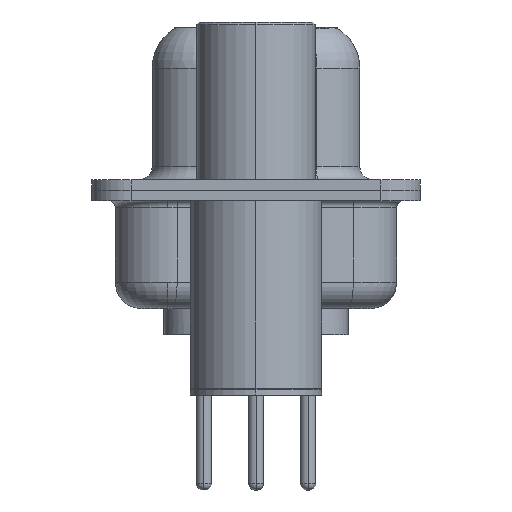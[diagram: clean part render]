
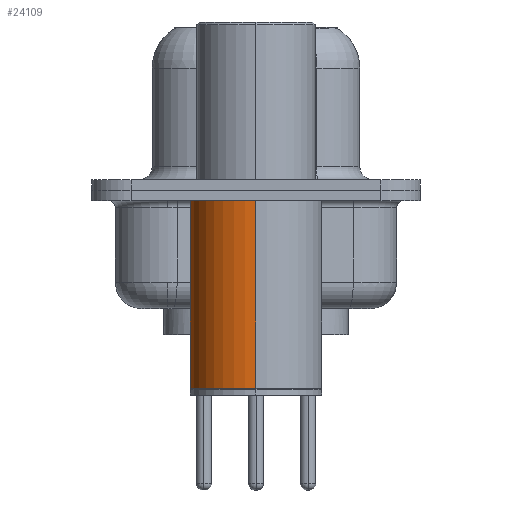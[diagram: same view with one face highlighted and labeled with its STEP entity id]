
A CAD part, left-side view. The second image highlights one B-rep face of the part: STEP entity #24109.
In plain terms, the highlighted cylindrical face has radius 2.5 mm (diameter 5 mm), a partial arc.
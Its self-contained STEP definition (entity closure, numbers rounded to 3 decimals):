
#884 = EDGE_CURVE ( 'NONE', #31840, #3143, #14207, .T. ) ;
#1985 = ORIENTED_EDGE ( 'NONE', *, *, #25627, .T. ) ;
#2144 = VECTOR ( 'NONE', #2211, 1000. ) ;
#2211 = DIRECTION ( 'NONE',  ( 0., 0., 1. ) ) ;
#2372 = CARTESIAN_POINT ( 'NONE',  ( 2.5, 0., -7.525 ) ) ;
#3133 = VERTEX_POINT ( 'NONE', #2372 ) ;
#3143 = VERTEX_POINT ( 'NONE', #9293 ) ;
#4476 = DIRECTION ( 'NONE',  ( 1., 0., 0. ) ) ;
#4681 = DIRECTION ( 'NONE',  ( 1., 0., 0. ) ) ;
#7288 = VERTEX_POINT ( 'NONE', #30706 ) ;
#7752 = ORIENTED_EDGE ( 'NONE', *, *, #14204, .F. ) ;
#8628 = LINE ( 'NONE', #18679, #12367 ) ;
#9293 = CARTESIAN_POINT ( 'NONE',  ( -2.5, 0., -0.4 ) ) ;
#11117 = CARTESIAN_POINT ( 'NONE',  ( 0., 0., 0.581 ) ) ;
#12092 = DIRECTION ( 'NONE',  ( 0., 0., 1. ) ) ;
#12190 = CIRCLE ( 'NONE', #21144, 2.5 ) ;
#12367 = VECTOR ( 'NONE', #31345, 1000. ) ;
#12710 = AXIS2_PLACEMENT_3D ( 'NONE', #11117, #24132, #16705 ) ;
#13914 = CYLINDRICAL_SURFACE ( 'NONE', #12710, 2.5 ) ;
#14204 = EDGE_CURVE ( 'NONE', #3133, #31840, #27725, .T. ) ;
#14207 = CIRCLE ( 'NONE', #16828, 2.5 ) ;
#16705 = DIRECTION ( 'NONE',  ( 1., 0., 0. ) ) ;
#16828 = AXIS2_PLACEMENT_3D ( 'NONE', #21594, #22099, #4476 ) ;
#18679 = CARTESIAN_POINT ( 'NONE',  ( -2.5, 0., 0.581 ) ) ;
#21144 = AXIS2_PLACEMENT_3D ( 'NONE', #29698, #12092, #4681 ) ;
#21594 = CARTESIAN_POINT ( 'NONE',  ( 0., 0., -0.4 ) ) ;
#22099 = DIRECTION ( 'NONE',  ( 0., 0., 1. ) ) ;
#23635 = FACE_OUTER_BOUND ( 'NONE', #29499, .T. ) ;
#24109 = ADVANCED_FACE ( 'NONE', ( #23635 ), #13914, .T. ) ;
#24132 = DIRECTION ( 'NONE',  ( 0., 0., 1. ) ) ;
#24938 = CARTESIAN_POINT ( 'NONE',  ( 2.5, 0., 0.581 ) ) ;
#25627 = EDGE_CURVE ( 'NONE', #3133, #7288, #12190, .T. ) ;
#26473 = CARTESIAN_POINT ( 'NONE',  ( 2.5, 0., -0.4 ) ) ;
#26477 = ORIENTED_EDGE ( 'NONE', *, *, #30934, .T. ) ;
#27725 = LINE ( 'NONE', #24938, #2144 ) ;
#29499 = EDGE_LOOP ( 'NONE', ( #1985, #26477, #30570, #7752 ) ) ;
#29698 = CARTESIAN_POINT ( 'NONE',  ( 0., 0., -7.525 ) ) ;
#30570 = ORIENTED_EDGE ( 'NONE', *, *, #884, .F. ) ;
#30706 = CARTESIAN_POINT ( 'NONE',  ( -2.5, 0., -7.525 ) ) ;
#30934 = EDGE_CURVE ( 'NONE', #7288, #3143, #8628, .T. ) ;
#31345 = DIRECTION ( 'NONE',  ( 0., 0., 1. ) ) ;
#31840 = VERTEX_POINT ( 'NONE', #26473 ) ;
